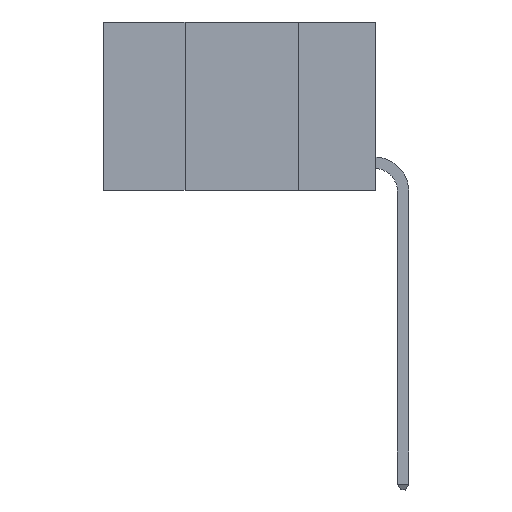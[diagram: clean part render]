
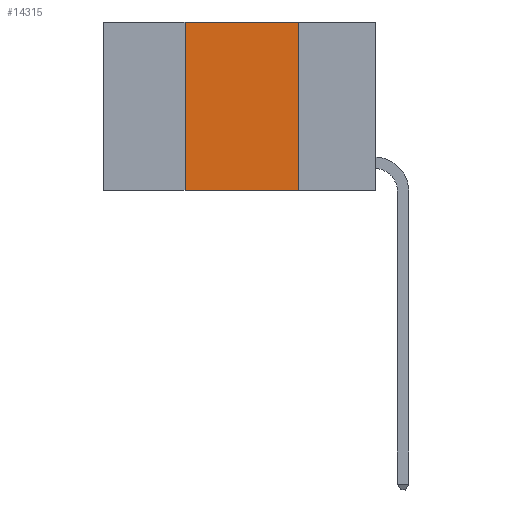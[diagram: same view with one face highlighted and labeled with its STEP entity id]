
A CAD part, left-side view. The second image highlights one B-rep face of the part: STEP entity #14315.
In plain terms, the highlighted planar face has unit normal (-1, 0, 0).
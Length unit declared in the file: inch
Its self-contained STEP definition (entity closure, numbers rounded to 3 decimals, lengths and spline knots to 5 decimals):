
#503 = AXIS2_PLACEMENT_3D ( 'NONE', #28431, #6453, #22051 ) ;
#1097 = LINE ( 'NONE', #17610, #7767 ) ;
#1352 = EDGE_LOOP ( 'NONE', ( #12387, #18316, #19709, #2553 ) ) ;
#1555 = EDGE_CURVE ( 'NONE', #12622, #4403, #1097, .T. ) ;
#2541 = LINE ( 'NONE', #26515, #26175 ) ;
#2553 = ORIENTED_EDGE ( 'NONE', *, *, #1555, .T. ) ;
#4403 = VERTEX_POINT ( 'NONE', #27741 ) ;
#5029 = FACE_OUTER_BOUND ( 'NONE', #1352, .T. ) ;
#6021 = VECTOR ( 'NONE', #12408, 39.37008 ) ;
#6453 = DIRECTION ( 'NONE',  ( 1., 0., 0. ) ) ;
#7427 = DIRECTION ( 'NONE',  ( 0., -1., 0. ) ) ;
#7767 = VECTOR ( 'NONE', #21958, 39.37008 ) ;
#7866 = CARTESIAN_POINT ( 'NONE',  ( 0., 0.42, 0. ) ) ;
#9665 = CARTESIAN_POINT ( 'NONE',  ( 0., 0.6, 0. ) ) ;
#11259 = VECTOR ( 'NONE', #7427, 39.37008 ) ;
#12387 = ORIENTED_EDGE ( 'NONE', *, *, #15676, .F. ) ;
#12408 = DIRECTION ( 'NONE',  ( 0., 0., 1. ) ) ;
#12622 = VERTEX_POINT ( 'NONE', #16105 ) ;
#13358 = DIRECTION ( 'NONE',  ( 0., 0., -1. ) ) ;
#14315 = ADVANCED_FACE ( 'NONE', ( #5029 ), #19845, .F. ) ;
#15323 = CARTESIAN_POINT ( 'NONE',  ( 0., 0.42, 0. ) ) ;
#15676 = EDGE_CURVE ( 'NONE', #19898, #4403, #2541, .T. ) ;
#16105 = CARTESIAN_POINT ( 'NONE',  ( 0., 0.42, -0.37 ) ) ;
#17610 = CARTESIAN_POINT ( 'NONE',  ( 0., 0.6, -0.37 ) ) ;
#18316 = ORIENTED_EDGE ( 'NONE', *, *, #26983, .F. ) ;
#19709 = ORIENTED_EDGE ( 'NONE', *, *, #25973, .F. ) ;
#19845 = PLANE ( 'NONE',  #503 ) ;
#19898 = VERTEX_POINT ( 'NONE', #21749 ) ;
#21749 = CARTESIAN_POINT ( 'NONE',  ( 0., 0.17, 0. ) ) ;
#21958 = DIRECTION ( 'NONE',  ( 0., -1., 0. ) ) ;
#22051 = DIRECTION ( 'NONE',  ( 0., 0., -1. ) ) ;
#23093 = LINE ( 'NONE', #9665, #11259 ) ;
#23795 = LINE ( 'NONE', #7866, #6021 ) ;
#24894 = VERTEX_POINT ( 'NONE', #15323 ) ;
#25973 = EDGE_CURVE ( 'NONE', #12622, #24894, #23795, .T. ) ;
#26175 = VECTOR ( 'NONE', #13358, 39.37008 ) ;
#26515 = CARTESIAN_POINT ( 'NONE',  ( 0., 0.17, 0. ) ) ;
#26983 = EDGE_CURVE ( 'NONE', #24894, #19898, #23093, .T. ) ;
#27741 = CARTESIAN_POINT ( 'NONE',  ( 0., 0.17, -0.37 ) ) ;
#28431 = CARTESIAN_POINT ( 'NONE',  ( 0., 0.6, 0. ) ) ;
